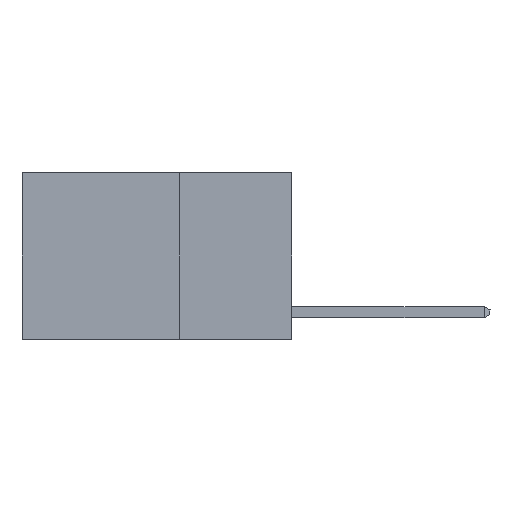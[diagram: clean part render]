
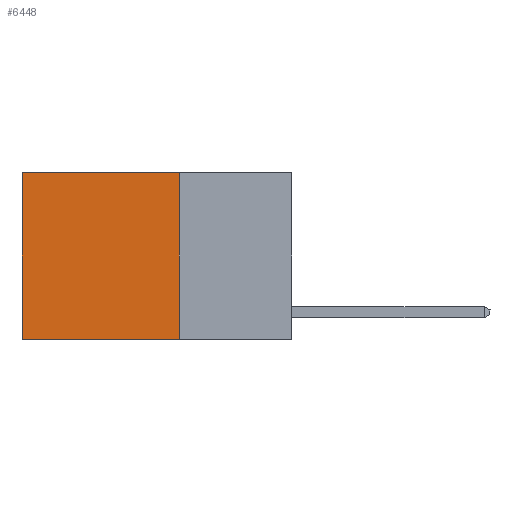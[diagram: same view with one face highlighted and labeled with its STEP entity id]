
A CAD part, left-side view. The second image highlights one B-rep face of the part: STEP entity #6448.
In plain terms, the highlighted planar face has unit normal (-1, 0, 0).
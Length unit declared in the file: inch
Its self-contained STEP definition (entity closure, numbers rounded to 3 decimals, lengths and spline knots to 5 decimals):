
#197 = CARTESIAN_POINT ( 'NONE',  ( 0.2625, 0.25, -0.37 ) ) ;
#1347 = EDGE_CURVE ( 'NONE', #13651, #13062, #10026, .T. ) ;
#2087 = EDGE_CURVE ( 'NONE', #19969, #13651, #8785, .T. ) ;
#2663 = PLANE ( 'NONE',  #16394 ) ;
#2913 = ORIENTED_EDGE ( 'NONE', *, *, #2087, .T. ) ;
#3401 = CARTESIAN_POINT ( 'NONE',  ( 0.2625, 0.6, 0. ) ) ;
#4018 = DIRECTION ( 'NONE',  ( 0., 0., -1. ) ) ;
#4300 = DIRECTION ( 'NONE',  ( 1., 0., 0. ) ) ;
#4881 = CARTESIAN_POINT ( 'NONE',  ( 0.2625, 0.25, 0. ) ) ;
#6448 = ADVANCED_FACE ( 'NONE', ( #18552 ), #2663, .F. ) ;
#7226 = CARTESIAN_POINT ( 'NONE',  ( 0.2625, 0.25, 0. ) ) ;
#7642 = DIRECTION ( 'NONE',  ( 0., 1., 0. ) ) ;
#7705 = CARTESIAN_POINT ( 'NONE',  ( 0.2625, 0.25, 0. ) ) ;
#7882 = ORIENTED_EDGE ( 'NONE', *, *, #1347, .T. ) ;
#8785 = LINE ( 'NONE', #19928, #12439 ) ;
#9056 = ORIENTED_EDGE ( 'NONE', *, *, #13572, .F. ) ;
#9999 = ORIENTED_EDGE ( 'NONE', *, *, #10247, .F. ) ;
#10026 = LINE ( 'NONE', #10192, #13679 ) ;
#10192 = CARTESIAN_POINT ( 'NONE',  ( 0.2625, 0.6, 0. ) ) ;
#10247 = EDGE_CURVE ( 'NONE', #17883, #13062, #10692, .T. ) ;
#10692 = LINE ( 'NONE', #197, #15301 ) ;
#11039 = VECTOR ( 'NONE', #15581, 39.37008 ) ;
#11767 = LINE ( 'NONE', #7705, #11039 ) ;
#11812 = CARTESIAN_POINT ( 'NONE',  ( 0.2625, 0.25, -0.37 ) ) ;
#12439 = VECTOR ( 'NONE', #7642, 39.37008 ) ;
#12928 = EDGE_LOOP ( 'NONE', ( #7882, #9999, #9056, #2913 ) ) ;
#13062 = VERTEX_POINT ( 'NONE', #16356 ) ;
#13572 = EDGE_CURVE ( 'NONE', #19969, #17883, #11767, .T. ) ;
#13651 = VERTEX_POINT ( 'NONE', #3401 ) ;
#13679 = VECTOR ( 'NONE', #19586, 39.37008 ) ;
#14700 = DIRECTION ( 'NONE',  ( 0., 1., 0. ) ) ;
#15301 = VECTOR ( 'NONE', #14700, 39.37008 ) ;
#15581 = DIRECTION ( 'NONE',  ( 0., 0., -1. ) ) ;
#16356 = CARTESIAN_POINT ( 'NONE',  ( 0.2625, 0.6, -0.37 ) ) ;
#16394 = AXIS2_PLACEMENT_3D ( 'NONE', #7226, #4300, #4018 ) ;
#17883 = VERTEX_POINT ( 'NONE', #11812 ) ;
#18552 = FACE_OUTER_BOUND ( 'NONE', #12928, .T. ) ;
#19586 = DIRECTION ( 'NONE',  ( 0., 0., -1. ) ) ;
#19928 = CARTESIAN_POINT ( 'NONE',  ( 0.2625, 0.25, 0. ) ) ;
#19969 = VERTEX_POINT ( 'NONE', #4881 ) ;
